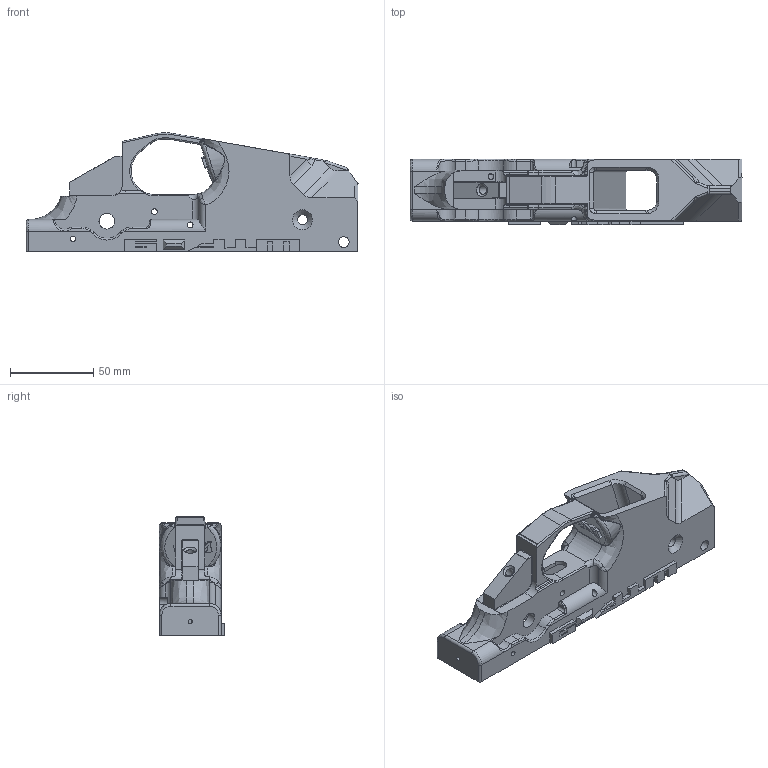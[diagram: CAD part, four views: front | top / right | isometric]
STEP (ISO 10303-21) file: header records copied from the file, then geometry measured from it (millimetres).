
FILE_DESCRIPTION (( 'STEP AP203' ), '1' );
FILE_NAME ('WTF-9MV_lower_receiver.STEP', '2020-06-09T21:36:59', ( '' ), ( '' ), 'SwSTEP 2.0', 'SolidWorks 2016', '' );
FILE_SCHEMA (( 'CONFIG_CONTROL_DESIGN' ));
Length unit declared in the file: millimetre
Products named in the file (1): WTF-9MV_lower_receiver
Bounding box: 199.47 x 39.37 x 71.26 mm (x, y, z)
Volume: 194835.4 mm3; surface area: 54841.4 mm2
Topology: 3 solids, 3 shells, 462 faces, 1261 edges, 790 vertices
Faces by surface type: plane 203, cylinder 140, bspline 116, cone 3
Full cylindrical faces by diameter (mm): 2.5 x1, 3 x1, 3.175 x3, 3.469 x4, 5.105 x1, 6 x1, 6.4 x2, 8 x1, 9.525 x2
Entity records: 22051 total; most frequent: CARTESIAN_POINT 11626, ORIENTED_EDGE 2430, DIRECTION 1689, EDGE_CURVE 1215, VERTEX_POINT 777, LINE 655, VECTOR 655, AXIS2_PLACEMENT_3D 517
